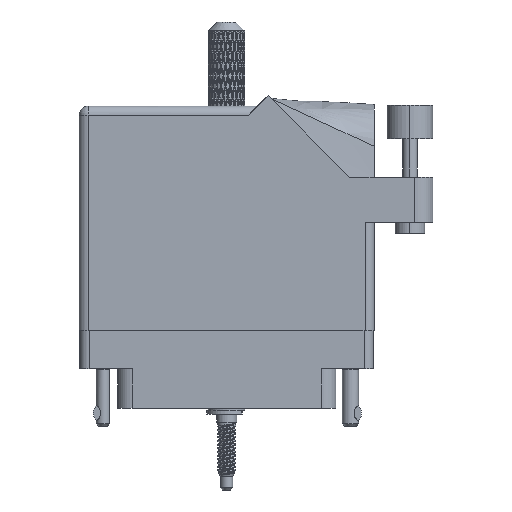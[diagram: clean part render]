
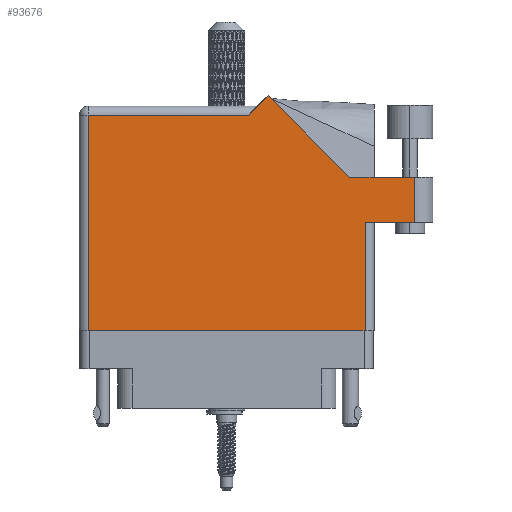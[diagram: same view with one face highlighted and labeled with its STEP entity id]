
A CAD part, front view. The second image highlights one B-rep face of the part: STEP entity #93676.
In plain terms, the highlighted face is planar.
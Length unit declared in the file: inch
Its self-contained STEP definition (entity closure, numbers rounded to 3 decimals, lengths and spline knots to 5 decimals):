
#403 = DIRECTION ( 'NONE',  ( -1., 0., 0. ) ) ;
#1756 = VERTEX_POINT ( 'NONE', #29237 ) ;
#3768 = EDGE_CURVE ( 'NONE', #1756, #61331, #65747, .T. ) ;
#3924 = CARTESIAN_POINT ( 'NONE',  ( 1.84442, 1.044, 0. ) ) ;
#4134 = VECTOR ( 'NONE', #68099, 39.37008 ) ;
#7095 = EDGE_CURVE ( 'NONE', #20123, #1756, #61028, .T. ) ;
#7295 = DIRECTION ( 'NONE',  ( 0., 1., 0. ) ) ;
#7390 = ORIENTED_EDGE ( 'NONE', *, *, #9952, .T. ) ;
#9952 = EDGE_CURVE ( 'NONE', #64673, #85089, #45579, .T. ) ;
#10751 = CARTESIAN_POINT ( 'NONE',  ( 1.217, 1.53, 0. ) ) ;
#10908 = EDGE_CURVE ( 'NONE', #41949, #60070, #16470, .T. ) ;
#11754 = AXIS2_PLACEMENT_3D ( 'NONE', #53272, #43673, #403 ) ;
#14607 = ORIENTED_EDGE ( 'NONE', *, *, #58162, .T. ) ;
#16470 = LINE ( 'NONE', #72081, #85243 ) ;
#16545 = CARTESIAN_POINT ( 'NONE',  ( 2.285, 1.044, 0. ) ) ;
#17616 = VECTOR ( 'NONE', #42740, 39.37008 ) ;
#18577 = ORIENTED_EDGE ( 'NONE', *, *, #3768, .T. ) ;
#19323 = DIRECTION ( 'NONE',  ( -1., 0., 0. ) ) ;
#20123 = VERTEX_POINT ( 'NONE', #47853 ) ;
#22734 = CARTESIAN_POINT ( 'NONE',  ( 1.948, 0., 0. ) ) ;
#25831 = CARTESIAN_POINT ( 'NONE',  ( 0., 0., 0. ) ) ;
#26183 = DIRECTION ( 'NONE',  ( 0., -1., 0. ) ) ;
#29216 = ORIENTED_EDGE ( 'NONE', *, *, #7095, .T. ) ;
#29237 = CARTESIAN_POINT ( 'NONE',  ( 2.285, 0.737, 0. ) ) ;
#29940 = VECTOR ( 'NONE', #7295, 39.37008 ) ;
#30657 = VECTOR ( 'NONE', #63490, 39.37008 ) ;
#34448 = DIRECTION ( 'NONE',  ( 0., 1., 0. ) ) ;
#38787 = CARTESIAN_POINT ( 'NONE',  ( 1.155, 1.468, 0. ) ) ;
#40877 = LINE ( 'NONE', #25831, #80797 ) ;
#40971 = LINE ( 'NONE', #100599, #93187 ) ;
#41949 = VERTEX_POINT ( 'NONE', #38787 ) ;
#42043 = VECTOR ( 'NONE', #34448, 39.37008 ) ;
#42740 = DIRECTION ( 'NONE',  ( -1., 0., 0. ) ) ;
#43673 = DIRECTION ( 'NONE',  ( 0., 0., -1. ) ) ;
#44420 = PLANE ( 'NONE',  #11754 ) ;
#45579 = LINE ( 'NONE', #59333, #4134 ) ;
#47853 = CARTESIAN_POINT ( 'NONE',  ( 1.948, 0.737, 0. ) ) ;
#52340 = CARTESIAN_POINT ( 'NONE',  ( 2.41, 1.044, 0. ) ) ;
#53272 = CARTESIAN_POINT ( 'NONE',  ( 0., 1.53, 0. ) ) ;
#54715 = DIRECTION ( 'NONE',  ( -0.707, -0.707, 0. ) ) ;
#57385 = EDGE_CURVE ( 'NONE', #61331, #64673, #105651, .T. ) ;
#58162 = EDGE_CURVE ( 'NONE', #58799, #63988, #40877, .T. ) ;
#58799 = VERTEX_POINT ( 'NONE', #69309 ) ;
#58853 = ORIENTED_EDGE ( 'NONE', *, *, #10908, .T. ) ;
#58944 = CARTESIAN_POINT ( 'NONE',  ( 0.062, 1.468, 0. ) ) ;
#59333 = CARTESIAN_POINT ( 'NONE',  ( 1.84442, 1.044, 0. ) ) ;
#60070 = VERTEX_POINT ( 'NONE', #58944 ) ;
#60669 = CARTESIAN_POINT ( 'NONE',  ( 1.948, 0.737, 0. ) ) ;
#61028 = LINE ( 'NONE', #88428, #30657 ) ;
#61331 = VERTEX_POINT ( 'NONE', #86131 ) ;
#63490 = DIRECTION ( 'NONE',  ( 1., 0., 0. ) ) ;
#63988 = VERTEX_POINT ( 'NONE', #22734 ) ;
#64673 = VERTEX_POINT ( 'NONE', #3924 ) ;
#65747 = LINE ( 'NONE', #16545, #29940 ) ;
#67845 = LINE ( 'NONE', #10751, #77628 ) ;
#68099 = DIRECTION ( 'NONE',  ( -0.707, 0.707, 0. ) ) ;
#69309 = CARTESIAN_POINT ( 'NONE',  ( 0.062, 0., 0. ) ) ;
#72081 = CARTESIAN_POINT ( 'NONE',  ( 0., 1.468, 0. ) ) ;
#77628 = VECTOR ( 'NONE', #54715, 39.37008 ) ;
#80554 = EDGE_LOOP ( 'NONE', ( #29216, #18577, #112086, #7390, #94633, #58853, #91377, #14607, #95865 ) ) ;
#80797 = VECTOR ( 'NONE', #93288, 39.37008 ) ;
#85089 = VERTEX_POINT ( 'NONE', #87249 ) ;
#85243 = VECTOR ( 'NONE', #19323, 39.37008 ) ;
#86131 = CARTESIAN_POINT ( 'NONE',  ( 2.285, 1.044, 0. ) ) ;
#87249 = CARTESIAN_POINT ( 'NONE',  ( 1.28771, 1.60071, 0. ) ) ;
#88428 = CARTESIAN_POINT ( 'NONE',  ( 2.01, 0.737, 0. ) ) ;
#91377 = ORIENTED_EDGE ( 'NONE', *, *, #106735, .T. ) ;
#93187 = VECTOR ( 'NONE', #26183, 39.37008 ) ;
#93288 = DIRECTION ( 'NONE',  ( 1., 0., 0. ) ) ;
#93676 = ADVANCED_FACE ( 'NONE', ( #112121 ), #44420, .F. ) ;
#94633 = ORIENTED_EDGE ( 'NONE', *, *, #111205, .T. ) ;
#95710 = LINE ( 'NONE', #60669, #42043 ) ;
#95865 = ORIENTED_EDGE ( 'NONE', *, *, #102258, .T. ) ;
#100599 = CARTESIAN_POINT ( 'NONE',  ( 0.062, 0., 0. ) ) ;
#102258 = EDGE_CURVE ( 'NONE', #63988, #20123, #95710, .T. ) ;
#105651 = LINE ( 'NONE', #52340, #17616 ) ;
#106735 = EDGE_CURVE ( 'NONE', #60070, #58799, #40971, .T. ) ;
#111205 = EDGE_CURVE ( 'NONE', #85089, #41949, #67845, .T. ) ;
#112086 = ORIENTED_EDGE ( 'NONE', *, *, #57385, .T. ) ;
#112121 = FACE_OUTER_BOUND ( 'NONE', #80554, .T. ) ;
